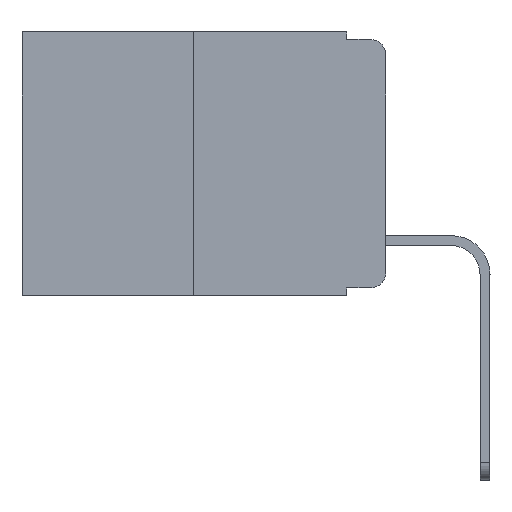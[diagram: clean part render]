
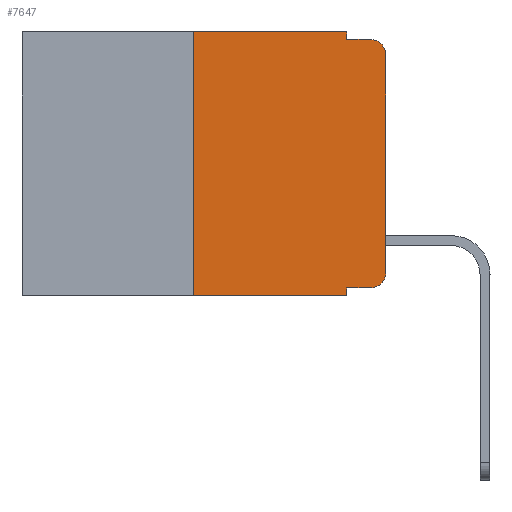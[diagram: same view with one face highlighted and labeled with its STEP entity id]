
A CAD part, left-side view. The second image highlights one B-rep face of the part: STEP entity #7647.
In plain terms, the highlighted planar face has unit normal (-1, 0, 0).
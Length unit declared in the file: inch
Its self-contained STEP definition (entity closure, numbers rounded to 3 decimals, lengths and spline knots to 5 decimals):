
#80 = ORIENTED_EDGE ( 'NONE', *, *, #2067, .F. ) ;
#142 = FACE_OUTER_BOUND ( 'NONE', #2467, .T. ) ;
#417 = CARTESIAN_POINT ( 'NONE',  ( 0., 0.051, 0. ) ) ;
#504 = EDGE_CURVE ( 'NONE', #506, #6659, #6852, .T. ) ;
#506 = VERTEX_POINT ( 'NONE', #6895 ) ;
#816 = CARTESIAN_POINT ( 'NONE',  ( 0., 0., 0. ) ) ;
#959 = LINE ( 'NONE', #816, #7897 ) ;
#1208 = CARTESIAN_POINT ( 'NONE',  ( 0., 0.25, 0. ) ) ;
#1374 = ORIENTED_EDGE ( 'NONE', *, *, #7845, .T. ) ;
#1387 = VERTEX_POINT ( 'NONE', #7589 ) ;
#1558 = ORIENTED_EDGE ( 'NONE', *, *, #4348, .F. ) ;
#1628 = EDGE_CURVE ( 'NONE', #9937, #4943, #8287, .T. ) ;
#1959 = PLANE ( 'NONE',  #8017 ) ;
#2016 = CARTESIAN_POINT ( 'NONE',  ( 0., 0.02, -0.01 ) ) ;
#2067 = EDGE_CURVE ( 'NONE', #5476, #2858, #8679, .T. ) ;
#2132 = DIRECTION ( 'NONE',  ( 0., -1., 0. ) ) ;
#2247 = CARTESIAN_POINT ( 'NONE',  ( 0., 0.473, 0. ) ) ;
#2257 = DIRECTION ( 'NONE',  ( 0., 0., -1. ) ) ;
#2467 = EDGE_LOOP ( 'NONE', ( #5366, #10302, #7525, #4366, #7783, #80, #6530, #1558, #2729, #1374 ) ) ;
#2472 = LINE ( 'NONE', #4394, #7123 ) ;
#2729 = ORIENTED_EDGE ( 'NONE', *, *, #504, .T. ) ;
#2858 = VERTEX_POINT ( 'NONE', #6424 ) ;
#2880 = VERTEX_POINT ( 'NONE', #6281 ) ;
#3618 = DIRECTION ( 'NONE',  ( 0., 0., -1. ) ) ;
#3690 = CARTESIAN_POINT ( 'NONE',  ( 0., 0.473, 0. ) ) ;
#3721 = DIRECTION ( 'NONE',  ( 0., -1., 0. ) ) ;
#3725 = DIRECTION ( 'NONE',  ( 0., 0., 1. ) ) ;
#3787 = CARTESIAN_POINT ( 'NONE',  ( 0., 0., -0.03 ) ) ;
#3966 = VECTOR ( 'NONE', #4479, 39.37008 ) ;
#4348 = EDGE_CURVE ( 'NONE', #506, #1387, #9132, .T. ) ;
#4366 = ORIENTED_EDGE ( 'NONE', *, *, #9215, .F. ) ;
#4394 = CARTESIAN_POINT ( 'NONE',  ( 0., 0.051, 0. ) ) ;
#4479 = DIRECTION ( 'NONE',  ( 0., -1., 0. ) ) ;
#4858 = DIRECTION ( 'NONE',  ( 0., 0., -1. ) ) ;
#4943 = VERTEX_POINT ( 'NONE', #2016 ) ;
#5366 = ORIENTED_EDGE ( 'NONE', *, *, #9820, .T. ) ;
#5395 = LINE ( 'NONE', #2247, #8693 ) ;
#5476 = VERTEX_POINT ( 'NONE', #7445 ) ;
#5907 = CARTESIAN_POINT ( 'NONE',  ( 0., 0.02, -0.313 ) ) ;
#6082 = LINE ( 'NONE', #10769, #6740 ) ;
#6119 = CARTESIAN_POINT ( 'NONE',  ( 0., 0.051, -0.333 ) ) ;
#6281 = CARTESIAN_POINT ( 'NONE',  ( 0., 0.051, -0.01 ) ) ;
#6312 = LINE ( 'NONE', #9661, #7105 ) ;
#6348 = VECTOR ( 'NONE', #4858, 39.37008 ) ;
#6403 = CARTESIAN_POINT ( 'NONE',  ( 0., 0.051, 0. ) ) ;
#6424 = CARTESIAN_POINT ( 'NONE',  ( 0., 0.25, 0. ) ) ;
#6472 = AXIS2_PLACEMENT_3D ( 'NONE', #5907, #6677, #7482 ) ;
#6530 = ORIENTED_EDGE ( 'NONE', *, *, #9206, .T. ) ;
#6659 = VERTEX_POINT ( 'NONE', #9105 ) ;
#6677 = DIRECTION ( 'NONE',  ( -1., 0., 0. ) ) ;
#6740 = VECTOR ( 'NONE', #8363, 39.37008 ) ;
#6852 = LINE ( 'NONE', #6119, #3966 ) ;
#6895 = CARTESIAN_POINT ( 'NONE',  ( 0., 0.051, -0.333 ) ) ;
#7105 = VECTOR ( 'NONE', #2132, 39.37008 ) ;
#7123 = VECTOR ( 'NONE', #9284, 39.37008 ) ;
#7445 = CARTESIAN_POINT ( 'NONE',  ( 0., 0.25, -0.343 ) ) ;
#7482 = DIRECTION ( 'NONE',  ( 0., 0., -1. ) ) ;
#7525 = ORIENTED_EDGE ( 'NONE', *, *, #9961, .F. ) ;
#7589 = CARTESIAN_POINT ( 'NONE',  ( 0., 0.051, -0.343 ) ) ;
#7647 = ADVANCED_FACE ( 'NONE', ( #142 ), #1959, .F. ) ;
#7730 = CIRCLE ( 'NONE', #6472, 0.02 ) ;
#7783 = ORIENTED_EDGE ( 'NONE', *, *, #10815, .F. ) ;
#7845 = EDGE_CURVE ( 'NONE', #6659, #9399, #7730, .T. ) ;
#7897 = VECTOR ( 'NONE', #9325, 39.37008 ) ;
#8017 = AXIS2_PLACEMENT_3D ( 'NONE', #3690, #8653, #3618 ) ;
#8273 = AXIS2_PLACEMENT_3D ( 'NONE', #10617, #9893, #2257 ) ;
#8287 = CIRCLE ( 'NONE', #8273, 0.02 ) ;
#8363 = DIRECTION ( 'NONE',  ( 0., -1., 0. ) ) ;
#8653 = DIRECTION ( 'NONE',  ( 1., 0., 0. ) ) ;
#8679 = LINE ( 'NONE', #1208, #9208 ) ;
#8693 = VECTOR ( 'NONE', #3721, 39.37008 ) ;
#8765 = CARTESIAN_POINT ( 'NONE',  ( 0., 0., -0.313 ) ) ;
#9105 = CARTESIAN_POINT ( 'NONE',  ( 0., 0.02, -0.333 ) ) ;
#9132 = LINE ( 'NONE', #6403, #6348 ) ;
#9206 = EDGE_CURVE ( 'NONE', #5476, #1387, #6082, .T. ) ;
#9208 = VECTOR ( 'NONE', #3725, 39.37008 ) ;
#9215 = EDGE_CURVE ( 'NONE', #9389, #2880, #2472, .T. ) ;
#9284 = DIRECTION ( 'NONE',  ( 0., 0., -1. ) ) ;
#9325 = DIRECTION ( 'NONE',  ( 0., 0., 1. ) ) ;
#9389 = VERTEX_POINT ( 'NONE', #417 ) ;
#9399 = VERTEX_POINT ( 'NONE', #8765 ) ;
#9661 = CARTESIAN_POINT ( 'NONE',  ( 0., 0.051, -0.01 ) ) ;
#9820 = EDGE_CURVE ( 'NONE', #9399, #9937, #959, .T. ) ;
#9893 = DIRECTION ( 'NONE',  ( -1., 0., 0. ) ) ;
#9937 = VERTEX_POINT ( 'NONE', #3787 ) ;
#9961 = EDGE_CURVE ( 'NONE', #2880, #4943, #6312, .T. ) ;
#10302 = ORIENTED_EDGE ( 'NONE', *, *, #1628, .T. ) ;
#10617 = CARTESIAN_POINT ( 'NONE',  ( 0., 0.02, -0.03 ) ) ;
#10769 = CARTESIAN_POINT ( 'NONE',  ( 0., 0.473, -0.343 ) ) ;
#10815 = EDGE_CURVE ( 'NONE', #2858, #9389, #5395, .T. ) ;
